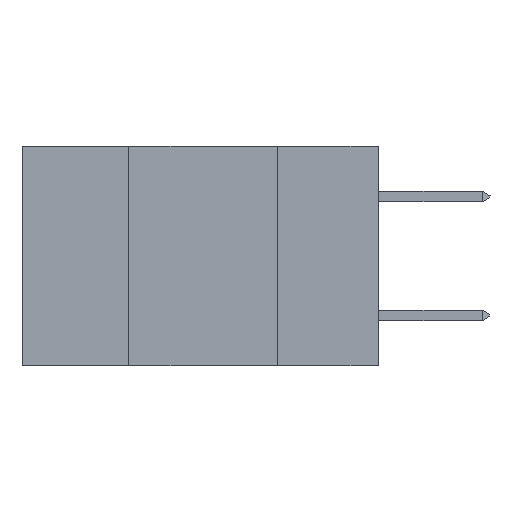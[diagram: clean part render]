
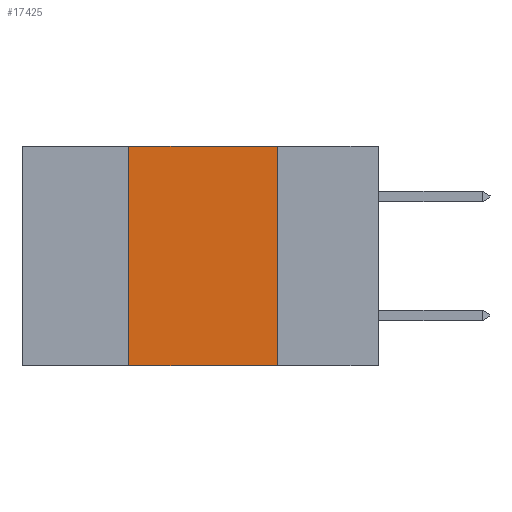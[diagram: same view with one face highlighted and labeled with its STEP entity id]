
A CAD part, left-side view. The second image highlights one B-rep face of the part: STEP entity #17425.
In plain terms, the highlighted planar face has unit normal (-1, 0, 0).
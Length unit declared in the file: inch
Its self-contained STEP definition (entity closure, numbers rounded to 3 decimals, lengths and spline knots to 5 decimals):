
#651 = CARTESIAN_POINT ( 'NONE',  ( 0., 0.6, 0. ) ) ;
#728 = CARTESIAN_POINT ( 'NONE',  ( 0., 0.6, -0.37 ) ) ;
#2624 = VERTEX_POINT ( 'NONE', #7177 ) ;
#3744 = EDGE_LOOP ( 'NONE', ( #11515, #8129, #19771, #10887 ) ) ;
#4239 = VERTEX_POINT ( 'NONE', #5601 ) ;
#4280 = DIRECTION ( 'NONE',  ( 0., 0., -1. ) ) ;
#5601 = CARTESIAN_POINT ( 'NONE',  ( 0., 0.42, -0.37 ) ) ;
#5705 = VECTOR ( 'NONE', #17884, 39.37008 ) ;
#6271 = LINE ( 'NONE', #10684, #19685 ) ;
#6372 = DIRECTION ( 'NONE',  ( 0., 0., 1. ) ) ;
#6596 = LINE ( 'NONE', #11503, #5705 ) ;
#7177 = CARTESIAN_POINT ( 'NONE',  ( 0., 0.42, 0. ) ) ;
#7252 = LINE ( 'NONE', #728, #10948 ) ;
#7427 = VERTEX_POINT ( 'NONE', #18850 ) ;
#8129 = ORIENTED_EDGE ( 'NONE', *, *, #18546, .F. ) ;
#8485 = DIRECTION ( 'NONE',  ( 0., -1., 0. ) ) ;
#8694 = PLANE ( 'NONE',  #9608 ) ;
#9608 = AXIS2_PLACEMENT_3D ( 'NONE', #651, #11559, #14916 ) ;
#10005 = EDGE_CURVE ( 'NONE', #4239, #17523, #7252, .T. ) ;
#10684 = CARTESIAN_POINT ( 'NONE',  ( 0., 0.42, -0.37 ) ) ;
#10887 = ORIENTED_EDGE ( 'NONE', *, *, #10005, .T. ) ;
#10948 = VECTOR ( 'NONE', #8485, 39.37008 ) ;
#11503 = CARTESIAN_POINT ( 'NONE',  ( 0., 0.6, 0. ) ) ;
#11515 = ORIENTED_EDGE ( 'NONE', *, *, #12053, .F. ) ;
#11559 = DIRECTION ( 'NONE',  ( 1., 0., 0. ) ) ;
#11987 = VECTOR ( 'NONE', #4280, 39.37008 ) ;
#12037 = LINE ( 'NONE', #16805, #11987 ) ;
#12053 = EDGE_CURVE ( 'NONE', #7427, #17523, #12037, .T. ) ;
#14916 = DIRECTION ( 'NONE',  ( 0., 0., -1. ) ) ;
#16413 = FACE_OUTER_BOUND ( 'NONE', #3744, .T. ) ;
#16805 = CARTESIAN_POINT ( 'NONE',  ( 0., 0.17, -0.37 ) ) ;
#16923 = CARTESIAN_POINT ( 'NONE',  ( 0., 0.17, -0.37 ) ) ;
#17425 = ADVANCED_FACE ( 'NONE', ( #16413 ), #8694, .F. ) ;
#17523 = VERTEX_POINT ( 'NONE', #16923 ) ;
#17884 = DIRECTION ( 'NONE',  ( 0., -1., 0. ) ) ;
#18546 = EDGE_CURVE ( 'NONE', #2624, #7427, #6596, .T. ) ;
#18812 = EDGE_CURVE ( 'NONE', #4239, #2624, #6271, .T. ) ;
#18850 = CARTESIAN_POINT ( 'NONE',  ( 0., 0.17, 0. ) ) ;
#19685 = VECTOR ( 'NONE', #6372, 39.37008 ) ;
#19771 = ORIENTED_EDGE ( 'NONE', *, *, #18812, .F. ) ;
